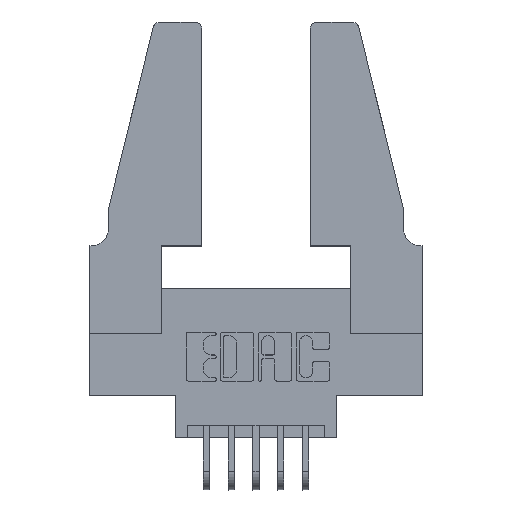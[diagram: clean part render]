
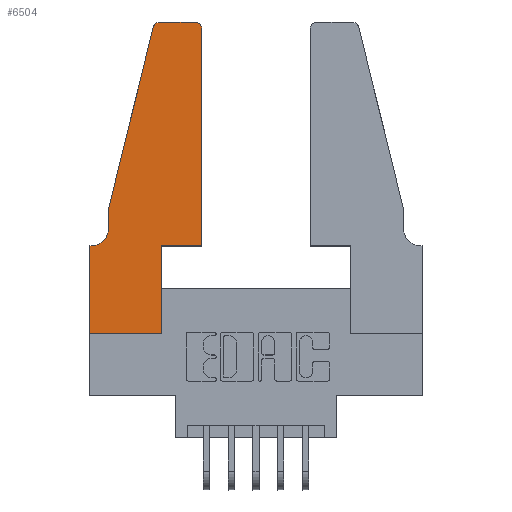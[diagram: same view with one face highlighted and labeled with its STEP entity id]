
A CAD part, top view. The second image highlights one B-rep face of the part: STEP entity #6504.
In plain terms, the highlighted planar face has unit normal (0, 0, 1).
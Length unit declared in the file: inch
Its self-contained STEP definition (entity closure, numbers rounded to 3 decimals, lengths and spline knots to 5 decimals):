
#559 = ORIENTED_EDGE ( 'NONE', *, *, #2441, .T. ) ;
#579 = VECTOR ( 'NONE', #4121, 39.37008 ) ;
#814 = CARTESIAN_POINT ( 'NONE',  ( 0.0755, 0.35, 0.37 ) ) ;
#834 = CARTESIAN_POINT ( 'NONE',  ( 0.0755, 0.42, 0.37 ) ) ;
#1073 = VERTEX_POINT ( 'NONE', #2851 ) ;
#1078 = EDGE_CURVE ( 'NONE', #10838, #4443, #6752, .T. ) ;
#1344 = VECTOR ( 'NONE', #5895, 39.37008 ) ;
#1418 = LINE ( 'NONE', #12254, #11646 ) ;
#1568 = ORIENTED_EDGE ( 'NONE', *, *, #5465, .T. ) ;
#1704 = DIRECTION ( 'NONE',  ( 0., -1., 0. ) ) ;
#1746 = LINE ( 'NONE', #12027, #9389 ) ;
#1948 = LINE ( 'NONE', #814, #7252 ) ;
#2037 = CARTESIAN_POINT ( 'NONE',  ( 0.2865, 0.35, 0.37 ) ) ;
#2281 = PLANE ( 'NONE',  #3573 ) ;
#2441 = EDGE_CURVE ( 'NONE', #2929, #11192, #1418, .T. ) ;
#2851 = CARTESIAN_POINT ( 'NONE',  ( 0., 0., 0.37 ) ) ;
#2878 = VECTOR ( 'NONE', #1704, 39.37008 ) ;
#2929 = VERTEX_POINT ( 'NONE', #6643 ) ;
#3098 = VERTEX_POINT ( 'NONE', #5705 ) ;
#3410 = CIRCLE ( 'NONE', #10865, 0.07 ) ;
#3573 = AXIS2_PLACEMENT_3D ( 'NONE', #4276, #11236, #5271 ) ;
#3649 = ORIENTED_EDGE ( 'NONE', *, *, #11435, .T. ) ;
#3692 = CARTESIAN_POINT ( 'NONE',  ( 0.284, 1.25, 0.37 ) ) ;
#3885 = EDGE_LOOP ( 'NONE', ( #559, #11505, #9438, #9473, #8618, #4926, #1568, #3649, #8700, #7358, #9004, #6390 ) ) ;
#4121 = DIRECTION ( 'NONE',  ( 1., 0., 0. ) ) ;
#4276 = CARTESIAN_POINT ( 'NONE',  ( 0., 0.35, 0.37 ) ) ;
#4443 = VERTEX_POINT ( 'NONE', #834 ) ;
#4663 = DIRECTION ( 'NONE',  ( 0., -1., 0. ) ) ;
#4840 = VECTOR ( 'NONE', #12231, 39.37008 ) ;
#4872 = FACE_OUTER_BOUND ( 'NONE', #3885, .T. ) ;
#4926 = ORIENTED_EDGE ( 'NONE', *, *, #5567, .T. ) ;
#5034 = DIRECTION ( 'NONE',  ( 0., 0., 1. ) ) ;
#5115 = DIRECTION ( 'NONE',  ( 1., 0., 0. ) ) ;
#5155 = LINE ( 'NONE', #11284, #4840 ) ;
#5254 = CARTESIAN_POINT ( 'NONE',  ( 0.0755, 0.5, 0.37 ) ) ;
#5271 = DIRECTION ( 'NONE',  ( 1., 0., 0. ) ) ;
#5465 = EDGE_CURVE ( 'NONE', #6689, #1073, #11131, .T. ) ;
#5567 = EDGE_CURVE ( 'NONE', #3098, #6689, #1948, .T. ) ;
#5639 = VECTOR ( 'NONE', #6276, 39.37008 ) ;
#5701 = DIRECTION ( 'NONE',  ( 0., 0., -1. ) ) ;
#5705 = CARTESIAN_POINT ( 'NONE',  ( 0.0055, 0.35, 0.37 ) ) ;
#5895 = DIRECTION ( 'NONE',  ( 0., 1., 0. ) ) ;
#5946 = DIRECTION ( 'NONE',  ( 0., 0., 1. ) ) ;
#5962 = LINE ( 'NONE', #5254, #5639 ) ;
#6115 = CARTESIAN_POINT ( 'NONE',  ( 0.0755, 0.5, 0.37 ) ) ;
#6176 = CARTESIAN_POINT ( 'NONE',  ( 0.0755, 0.5, 0.37 ) ) ;
#6276 = DIRECTION ( 'NONE',  ( -0.239, -0.971, 0. ) ) ;
#6327 = LINE ( 'NONE', #11818, #1344 ) ;
#6390 = ORIENTED_EDGE ( 'NONE', *, *, #12531, .T. ) ;
#6445 = VECTOR ( 'NONE', #4663, 39.37008 ) ;
#6504 = ADVANCED_FACE ( 'NONE', ( #4872 ), #2281, .T. ) ;
#6643 = CARTESIAN_POINT ( 'NONE',  ( 0.4205, 1.25, 0.37 ) ) ;
#6689 = VERTEX_POINT ( 'NONE', #10507 ) ;
#6752 = LINE ( 'NONE', #6176, #6445 ) ;
#6837 = CARTESIAN_POINT ( 'NONE',  ( 0.25487, 1.22718, 0.37 ) ) ;
#7090 = EDGE_CURVE ( 'NONE', #7467, #10838, #5962, .T. ) ;
#7147 = AXIS2_PLACEMENT_3D ( 'NONE', #11003, #5034, #11952 ) ;
#7252 = VECTOR ( 'NONE', #9812, 39.37008 ) ;
#7358 = ORIENTED_EDGE ( 'NONE', *, *, #7704, .T. ) ;
#7467 = VERTEX_POINT ( 'NONE', #6837 ) ;
#7606 = VERTEX_POINT ( 'NONE', #2037 ) ;
#7704 = EDGE_CURVE ( 'NONE', #7606, #12297, #1746, .T. ) ;
#7821 = EDGE_CURVE ( 'NONE', #12297, #9944, #5155, .T. ) ;
#8187 = DIRECTION ( 'NONE',  ( -1., 0., 0. ) ) ;
#8540 = LINE ( 'NONE', #11098, #579 ) ;
#8618 = ORIENTED_EDGE ( 'NONE', *, *, #9345, .T. ) ;
#8700 = ORIENTED_EDGE ( 'NONE', *, *, #12489, .T. ) ;
#9004 = ORIENTED_EDGE ( 'NONE', *, *, #7821, .T. ) ;
#9173 = CIRCLE ( 'NONE', #7147, 0.03 ) ;
#9345 = EDGE_CURVE ( 'NONE', #4443, #3098, #3410, .T. ) ;
#9389 = VECTOR ( 'NONE', #5115, 39.37008 ) ;
#9438 = ORIENTED_EDGE ( 'NONE', *, *, #7090, .T. ) ;
#9473 = ORIENTED_EDGE ( 'NONE', *, *, #1078, .T. ) ;
#9812 = DIRECTION ( 'NONE',  ( -1., 0., 0. ) ) ;
#9944 = VERTEX_POINT ( 'NONE', #11500 ) ;
#10498 = CARTESIAN_POINT ( 'NONE',  ( 0.2865, 0., 0.37 ) ) ;
#10507 = CARTESIAN_POINT ( 'NONE',  ( 0., 0.35, 0.37 ) ) ;
#10806 = AXIS2_PLACEMENT_3D ( 'NONE', #11857, #5946, #12832 ) ;
#10838 = VERTEX_POINT ( 'NONE', #6115 ) ;
#10865 = AXIS2_PLACEMENT_3D ( 'NONE', #11632, #5701, #12597 ) ;
#10982 = CIRCLE ( 'NONE', #10806, 0.03 ) ;
#11003 = CARTESIAN_POINT ( 'NONE',  ( 0.284, 1.22, 0.37 ) ) ;
#11098 = CARTESIAN_POINT ( 'NONE',  ( 0., 0., 0.37 ) ) ;
#11131 = LINE ( 'NONE', #11580, #2878 ) ;
#11192 = VERTEX_POINT ( 'NONE', #3692 ) ;
#11236 = DIRECTION ( 'NONE',  ( 0., 0., 1. ) ) ;
#11284 = CARTESIAN_POINT ( 'NONE',  ( 0.4505, 0.35, 0.37 ) ) ;
#11391 = EDGE_CURVE ( 'NONE', #11192, #7467, #9173, .T. ) ;
#11435 = EDGE_CURVE ( 'NONE', #1073, #11754, #8540, .T. ) ;
#11500 = CARTESIAN_POINT ( 'NONE',  ( 0.4505, 1.22, 0.37 ) ) ;
#11505 = ORIENTED_EDGE ( 'NONE', *, *, #11391, .T. ) ;
#11580 = CARTESIAN_POINT ( 'NONE',  ( 0., 0., 0.37 ) ) ;
#11632 = CARTESIAN_POINT ( 'NONE',  ( 0.0055, 0.42, 0.37 ) ) ;
#11646 = VECTOR ( 'NONE', #8187, 39.37008 ) ;
#11754 = VERTEX_POINT ( 'NONE', #10498 ) ;
#11818 = CARTESIAN_POINT ( 'NONE',  ( 0.2865, 0.35, 0.37 ) ) ;
#11857 = CARTESIAN_POINT ( 'NONE',  ( 0.4205, 1.22, 0.37 ) ) ;
#11952 = DIRECTION ( 'NONE',  ( 1., 0., 0. ) ) ;
#12027 = CARTESIAN_POINT ( 'NONE',  ( 0.4505, 0.35, 0.37 ) ) ;
#12231 = DIRECTION ( 'NONE',  ( 0., 1., 0. ) ) ;
#12254 = CARTESIAN_POINT ( 'NONE',  ( 0.2605, 1.25, 0.37 ) ) ;
#12297 = VERTEX_POINT ( 'NONE', #12408 ) ;
#12408 = CARTESIAN_POINT ( 'NONE',  ( 0.4505, 0.35, 0.37 ) ) ;
#12489 = EDGE_CURVE ( 'NONE', #11754, #7606, #6327, .T. ) ;
#12531 = EDGE_CURVE ( 'NONE', #9944, #2929, #10982, .T. ) ;
#12597 = DIRECTION ( 'NONE',  ( -1., 0., 0. ) ) ;
#12832 = DIRECTION ( 'NONE',  ( 1., 0., 0. ) ) ;
